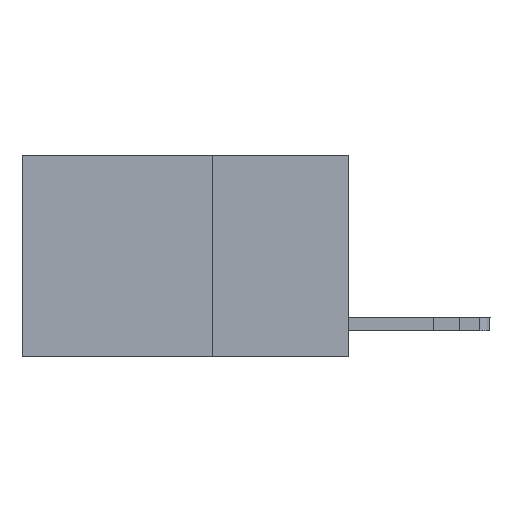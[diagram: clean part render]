
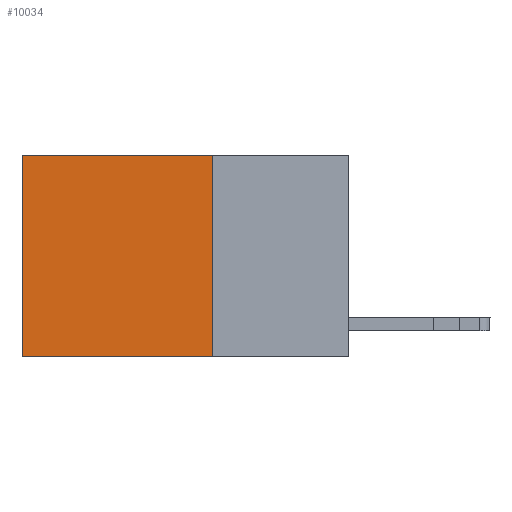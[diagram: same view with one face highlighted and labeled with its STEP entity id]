
A CAD part, left-side view. The second image highlights one B-rep face of the part: STEP entity #10034.
In plain terms, the highlighted planar face has unit normal (-1, 0, 0).
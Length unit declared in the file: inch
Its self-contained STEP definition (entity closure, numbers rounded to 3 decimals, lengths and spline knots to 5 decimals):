
#91 = VECTOR ( 'NONE', #4115, 39.37008 ) ;
#181 = EDGE_CURVE ( 'NONE', #4764, #10865, #6523, .T. ) ;
#664 = EDGE_CURVE ( 'NONE', #7306, #4764, #8537, .T. ) ;
#821 = DIRECTION ( 'NONE',  ( 0., 0., -1. ) ) ;
#1734 = CARTESIAN_POINT ( 'NONE',  ( 0.2625, 0.6, 0. ) ) ;
#2561 = EDGE_LOOP ( 'NONE', ( #7446, #10975, #3666, #3448 ) ) ;
#2733 = FACE_OUTER_BOUND ( 'NONE', #2561, .T. ) ;
#3248 = CARTESIAN_POINT ( 'NONE',  ( 0.2625, 0.25, -0.37 ) ) ;
#3448 = ORIENTED_EDGE ( 'NONE', *, *, #12842, .T. ) ;
#3666 = ORIENTED_EDGE ( 'NONE', *, *, #664, .F. ) ;
#3857 = VECTOR ( 'NONE', #12917, 39.37008 ) ;
#4115 = DIRECTION ( 'NONE',  ( 0., 0., -1. ) ) ;
#4195 = DIRECTION ( 'NONE',  ( 0., 1., 0. ) ) ;
#4764 = VERTEX_POINT ( 'NONE', #3248 ) ;
#5129 = DIRECTION ( 'NONE',  ( 1., 0., 0. ) ) ;
#5678 = LINE ( 'NONE', #8798, #3857 ) ;
#5978 = LINE ( 'NONE', #10126, #7496 ) ;
#6174 = CARTESIAN_POINT ( 'NONE',  ( 0.2625, 0.25, 0. ) ) ;
#6345 = PLANE ( 'NONE',  #11807 ) ;
#6523 = LINE ( 'NONE', #9125, #8310 ) ;
#7273 = DIRECTION ( 'NONE',  ( 0., 0., -1. ) ) ;
#7306 = VERTEX_POINT ( 'NONE', #12571 ) ;
#7446 = ORIENTED_EDGE ( 'NONE', *, *, #11980, .T. ) ;
#7496 = VECTOR ( 'NONE', #821, 39.37008 ) ;
#8310 = VECTOR ( 'NONE', #4195, 39.37008 ) ;
#8380 = VERTEX_POINT ( 'NONE', #1734 ) ;
#8537 = LINE ( 'NONE', #6174, #91 ) ;
#8798 = CARTESIAN_POINT ( 'NONE',  ( 0.2625, 0.25, 0. ) ) ;
#8834 = CARTESIAN_POINT ( 'NONE',  ( 0.2625, 0.6, -0.37 ) ) ;
#9125 = CARTESIAN_POINT ( 'NONE',  ( 0.2625, 0.25, -0.37 ) ) ;
#9252 = CARTESIAN_POINT ( 'NONE',  ( 0.2625, 0.25, 0. ) ) ;
#10034 = ADVANCED_FACE ( 'NONE', ( #2733 ), #6345, .F. ) ;
#10126 = CARTESIAN_POINT ( 'NONE',  ( 0.2625, 0.6, 0. ) ) ;
#10865 = VERTEX_POINT ( 'NONE', #8834 ) ;
#10975 = ORIENTED_EDGE ( 'NONE', *, *, #181, .F. ) ;
#11807 = AXIS2_PLACEMENT_3D ( 'NONE', #9252, #5129, #7273 ) ;
#11980 = EDGE_CURVE ( 'NONE', #8380, #10865, #5978, .T. ) ;
#12571 = CARTESIAN_POINT ( 'NONE',  ( 0.2625, 0.25, 0. ) ) ;
#12842 = EDGE_CURVE ( 'NONE', #7306, #8380, #5678, .T. ) ;
#12917 = DIRECTION ( 'NONE',  ( 0., 1., 0. ) ) ;
